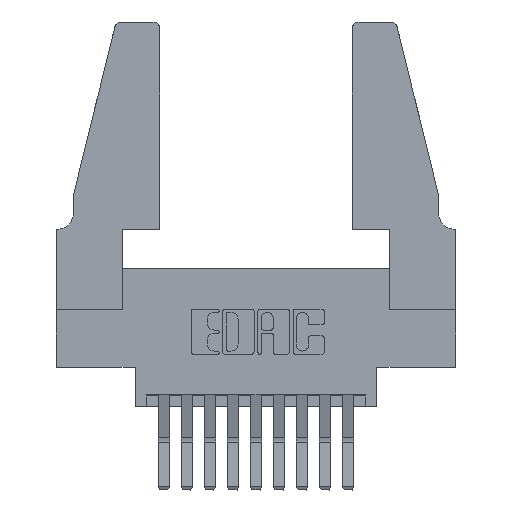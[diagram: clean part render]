
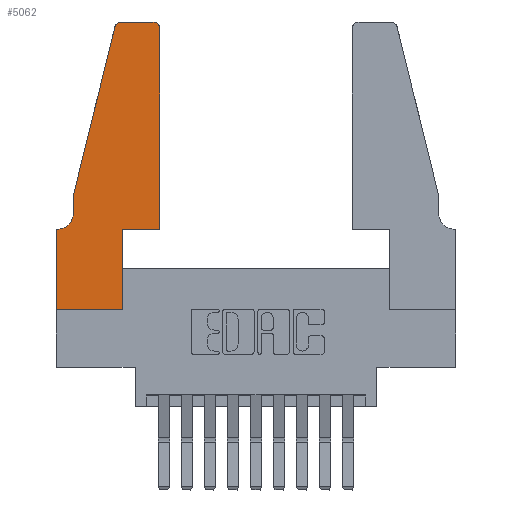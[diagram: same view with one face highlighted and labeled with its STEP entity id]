
A CAD part, top view. The second image highlights one B-rep face of the part: STEP entity #5062.
In plain terms, the highlighted planar face has unit normal (0, 0, 1).
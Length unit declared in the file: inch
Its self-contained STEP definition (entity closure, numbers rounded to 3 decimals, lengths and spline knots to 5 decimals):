
#61 = AXIS2_PLACEMENT_3D ( 'NONE', #6640, #10992, #11939 ) ;
#110 = ORIENTED_EDGE ( 'NONE', *, *, #13428, .T. ) ;
#464 = DIRECTION ( 'NONE',  ( 0., 1., 0. ) ) ;
#845 = ORIENTED_EDGE ( 'NONE', *, *, #9583, .T. ) ;
#1036 = CARTESIAN_POINT ( 'NONE',  ( 0.0055, 0.42, 0.37 ) ) ;
#1110 = EDGE_LOOP ( 'NONE', ( #6121, #1744, #5124, #9569, #5238, #3129, #1194, #8651, #4640, #845, #6733, #110 ) ) ;
#1194 = ORIENTED_EDGE ( 'NONE', *, *, #10165, .T. ) ;
#1256 = CARTESIAN_POINT ( 'NONE',  ( 0., 0., 0.37 ) ) ;
#1313 = CARTESIAN_POINT ( 'NONE',  ( 0.4505, 0.35, 0.37 ) ) ;
#1463 = AXIS2_PLACEMENT_3D ( 'NONE', #3640, #5800, #13299 ) ;
#1637 = VECTOR ( 'NONE', #12115, 39.37008 ) ;
#1744 = ORIENTED_EDGE ( 'NONE', *, *, #10792, .T. ) ;
#2189 = CARTESIAN_POINT ( 'NONE',  ( 0.0755, 0.5, 0.37 ) ) ;
#2324 = EDGE_CURVE ( 'NONE', #12687, #2711, #10774, .T. ) ;
#2335 = EDGE_CURVE ( 'NONE', #9409, #13658, #10106, .T. ) ;
#2454 = CARTESIAN_POINT ( 'NONE',  ( 0.2865, 0.35, 0.37 ) ) ;
#2525 = CIRCLE ( 'NONE', #7911, 0.03 ) ;
#2711 = VERTEX_POINT ( 'NONE', #7676 ) ;
#3129 = ORIENTED_EDGE ( 'NONE', *, *, #11641, .T. ) ;
#3261 = VERTEX_POINT ( 'NONE', #6468 ) ;
#3296 = DIRECTION ( 'NONE',  ( 0., 0., -1. ) ) ;
#3479 = VERTEX_POINT ( 'NONE', #11869 ) ;
#3503 = VECTOR ( 'NONE', #12056, 39.37008 ) ;
#3532 = CARTESIAN_POINT ( 'NONE',  ( 0.4505, 0.35, 0.37 ) ) ;
#3640 = CARTESIAN_POINT ( 'NONE',  ( 0.284, 1.22, 0.37 ) ) ;
#3818 = CARTESIAN_POINT ( 'NONE',  ( 0.4505, 0.35, 0.37 ) ) ;
#4225 = CARTESIAN_POINT ( 'NONE',  ( 0.0755, 0.42, 0.37 ) ) ;
#4558 = LINE ( 'NONE', #8795, #6583 ) ;
#4640 = ORIENTED_EDGE ( 'NONE', *, *, #9043, .T. ) ;
#4679 = LINE ( 'NONE', #2454, #1637 ) ;
#4884 = CARTESIAN_POINT ( 'NONE',  ( 0.4205, 1.22, 0.37 ) ) ;
#5062 = ADVANCED_FACE ( 'NONE', ( #8545 ), #5610, .T. ) ;
#5122 = EDGE_CURVE ( 'NONE', #12976, #10231, #6663, .T. ) ;
#5124 = ORIENTED_EDGE ( 'NONE', *, *, #5122, .T. ) ;
#5217 = DIRECTION ( 'NONE',  ( -1., 0., 0. ) ) ;
#5238 = ORIENTED_EDGE ( 'NONE', *, *, #12448, .T. ) ;
#5433 = CIRCLE ( 'NONE', #12720, 0.07 ) ;
#5610 = PLANE ( 'NONE',  #61 ) ;
#5632 = VERTEX_POINT ( 'NONE', #10146 ) ;
#5800 = DIRECTION ( 'NONE',  ( 0., 0., 1. ) ) ;
#5951 = VECTOR ( 'NONE', #10779, 39.37008 ) ;
#6114 = LINE ( 'NONE', #1256, #5951 ) ;
#6121 = ORIENTED_EDGE ( 'NONE', *, *, #2324, .T. ) ;
#6124 = CIRCLE ( 'NONE', #1463, 0.03 ) ;
#6157 = VECTOR ( 'NONE', #10610, 39.37008 ) ;
#6208 = CARTESIAN_POINT ( 'NONE',  ( 0.0755, 0.35, 0.37 ) ) ;
#6466 = CARTESIAN_POINT ( 'NONE',  ( 0.4505, 1.22, 0.37 ) ) ;
#6468 = CARTESIAN_POINT ( 'NONE',  ( 0.2865, 0.35, 0.37 ) ) ;
#6583 = VECTOR ( 'NONE', #9809, 39.37008 ) ;
#6640 = CARTESIAN_POINT ( 'NONE',  ( 0., 0.35, 0.37 ) ) ;
#6663 = LINE ( 'NONE', #9822, #8190 ) ;
#6733 = ORIENTED_EDGE ( 'NONE', *, *, #2335, .T. ) ;
#6755 = VECTOR ( 'NONE', #10971, 39.37008 ) ;
#6899 = CARTESIAN_POINT ( 'NONE',  ( 0.2605, 1.25, 0.37 ) ) ;
#7253 = VECTOR ( 'NONE', #464, 39.37008 ) ;
#7426 = EDGE_CURVE ( 'NONE', #10231, #7655, #4558, .T. ) ;
#7655 = VERTEX_POINT ( 'NONE', #4225 ) ;
#7676 = CARTESIAN_POINT ( 'NONE',  ( 0.284, 1.25, 0.37 ) ) ;
#7911 = AXIS2_PLACEMENT_3D ( 'NONE', #4884, #13409, #10263 ) ;
#8190 = VECTOR ( 'NONE', #10897, 39.37008 ) ;
#8545 = FACE_OUTER_BOUND ( 'NONE', #1110, .T. ) ;
#8651 = ORIENTED_EDGE ( 'NONE', *, *, #11478, .T. ) ;
#8795 = CARTESIAN_POINT ( 'NONE',  ( 0.0755, 0.5, 0.37 ) ) ;
#9043 = EDGE_CURVE ( 'NONE', #13615, #3261, #4679, .T. ) ;
#9160 = VERTEX_POINT ( 'NONE', #12199 ) ;
#9409 = VERTEX_POINT ( 'NONE', #3818 ) ;
#9569 = ORIENTED_EDGE ( 'NONE', *, *, #7426, .T. ) ;
#9583 = EDGE_CURVE ( 'NONE', #3261, #9409, #12541, .T. ) ;
#9809 = DIRECTION ( 'NONE',  ( 0., -1., 0. ) ) ;
#9815 = VECTOR ( 'NONE', #5217, 39.37008 ) ;
#9822 = CARTESIAN_POINT ( 'NONE',  ( 0.0755, 0.5, 0.37 ) ) ;
#9949 = CARTESIAN_POINT ( 'NONE',  ( 0.4205, 1.25, 0.37 ) ) ;
#10106 = LINE ( 'NONE', #3532, #7253 ) ;
#10146 = CARTESIAN_POINT ( 'NONE',  ( 0., 0.35, 0.37 ) ) ;
#10165 = EDGE_CURVE ( 'NONE', #5632, #3479, #11334, .T. ) ;
#10231 = VERTEX_POINT ( 'NONE', #2189 ) ;
#10263 = DIRECTION ( 'NONE',  ( 1., 0., 0. ) ) ;
#10610 = DIRECTION ( 'NONE',  ( 0., -1., 0. ) ) ;
#10704 = DIRECTION ( 'NONE',  ( -1., 0., 0. ) ) ;
#10774 = LINE ( 'NONE', #6899, #6755 ) ;
#10779 = DIRECTION ( 'NONE',  ( 1., 0., 0. ) ) ;
#10792 = EDGE_CURVE ( 'NONE', #2711, #12976, #6124, .T. ) ;
#10897 = DIRECTION ( 'NONE',  ( -0.239, -0.971, 0. ) ) ;
#10971 = DIRECTION ( 'NONE',  ( -1., 0., 0. ) ) ;
#10992 = DIRECTION ( 'NONE',  ( 0., 0., 1. ) ) ;
#11334 = LINE ( 'NONE', #13806, #6157 ) ;
#11478 = EDGE_CURVE ( 'NONE', #3479, #13615, #6114, .T. ) ;
#11641 = EDGE_CURVE ( 'NONE', #9160, #5632, #13840, .T. ) ;
#11815 = CARTESIAN_POINT ( 'NONE',  ( 0.25487, 1.22718, 0.37 ) ) ;
#11869 = CARTESIAN_POINT ( 'NONE',  ( 0., 0., 0.37 ) ) ;
#11939 = DIRECTION ( 'NONE',  ( 1., 0., 0. ) ) ;
#12056 = DIRECTION ( 'NONE',  ( 1., 0., 0. ) ) ;
#12115 = DIRECTION ( 'NONE',  ( 0., 1., 0. ) ) ;
#12199 = CARTESIAN_POINT ( 'NONE',  ( 0.0055, 0.35, 0.37 ) ) ;
#12448 = EDGE_CURVE ( 'NONE', #7655, #9160, #5433, .T. ) ;
#12541 = LINE ( 'NONE', #1313, #3503 ) ;
#12651 = CARTESIAN_POINT ( 'NONE',  ( 0.2865, 0., 0.37 ) ) ;
#12687 = VERTEX_POINT ( 'NONE', #9949 ) ;
#12720 = AXIS2_PLACEMENT_3D ( 'NONE', #1036, #3296, #10704 ) ;
#12976 = VERTEX_POINT ( 'NONE', #11815 ) ;
#13299 = DIRECTION ( 'NONE',  ( 1., 0., 0. ) ) ;
#13409 = DIRECTION ( 'NONE',  ( 0., 0., 1. ) ) ;
#13428 = EDGE_CURVE ( 'NONE', #13658, #12687, #2525, .T. ) ;
#13615 = VERTEX_POINT ( 'NONE', #12651 ) ;
#13658 = VERTEX_POINT ( 'NONE', #6466 ) ;
#13806 = CARTESIAN_POINT ( 'NONE',  ( 0., 0., 0.37 ) ) ;
#13840 = LINE ( 'NONE', #6208, #9815 ) ;
